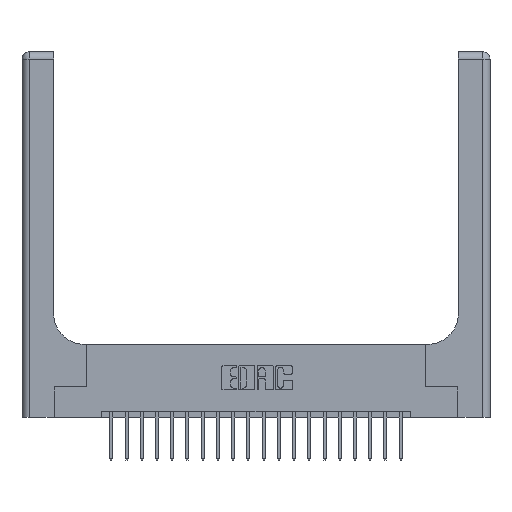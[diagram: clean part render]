
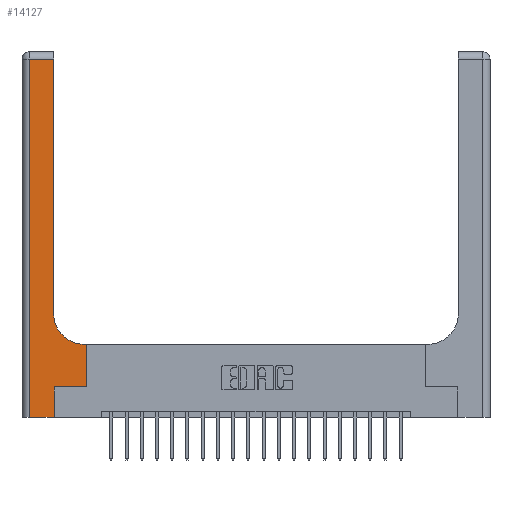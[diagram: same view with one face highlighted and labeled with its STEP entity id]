
A CAD part, top view. The second image highlights one B-rep face of the part: STEP entity #14127.
In plain terms, the highlighted planar face has unit normal (0, 0, 1).
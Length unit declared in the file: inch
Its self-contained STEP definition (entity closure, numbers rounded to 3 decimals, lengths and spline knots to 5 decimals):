
#174 = DIRECTION ( 'NONE',  ( 0., 0., -1. ) ) ;
#272 = ORIENTED_EDGE ( 'NONE', *, *, #4696, .T. ) ;
#410 = VECTOR ( 'NONE', #14561, 39.37008 ) ;
#433 = VERTEX_POINT ( 'NONE', #10053 ) ;
#831 = CARTESIAN_POINT ( 'NONE',  ( 0., 3., 0.37 ) ) ;
#858 = VERTEX_POINT ( 'NONE', #8702 ) ;
#1061 = ORIENTED_EDGE ( 'NONE', *, *, #18924, .T. ) ;
#1114 = CARTESIAN_POINT ( 'NONE',  ( 0.528, 0.25, 0.37 ) ) ;
#1406 = LINE ( 'NONE', #9498, #10198 ) ;
#1642 = EDGE_CURVE ( 'NONE', #13116, #433, #7675, .T. ) ;
#2088 = DIRECTION ( 'NONE',  ( 1., 0., 0. ) ) ;
#2135 = DIRECTION ( 'NONE',  ( 0., -1., 0. ) ) ;
#2728 = VECTOR ( 'NONE', #2088, 39.37008 ) ;
#2782 = VECTOR ( 'NONE', #2135, 39.37008 ) ;
#2784 = VECTOR ( 'NONE', #14777, 39.37008 ) ;
#2836 = CARTESIAN_POINT ( 'NONE',  ( 0.265, 0., 0.37 ) ) ;
#3030 = ORIENTED_EDGE ( 'NONE', *, *, #1642, .T. ) ;
#3148 = VECTOR ( 'NONE', #8522, 39.37008 ) ;
#3284 = VERTEX_POINT ( 'NONE', #2836 ) ;
#3618 = DIRECTION ( 'NONE',  ( -1., 0., 0. ) ) ;
#3716 = LINE ( 'NONE', #10381, #3148 ) ;
#3852 = DIRECTION ( 'NONE',  ( -1., 0., 0. ) ) ;
#4226 = EDGE_CURVE ( 'NONE', #858, #3284, #10407, .T. ) ;
#4638 = ORIENTED_EDGE ( 'NONE', *, *, #8889, .T. ) ;
#4696 = EDGE_CURVE ( 'NONE', #7292, #8135, #3716, .T. ) ;
#4708 = CARTESIAN_POINT ( 'NONE',  ( 0.26, 3., 0.37 ) ) ;
#4794 = CARTESIAN_POINT ( 'NONE',  ( 0.06, 2.94, 0.37 ) ) ;
#4883 = ORIENTED_EDGE ( 'NONE', *, *, #4226, .T. ) ;
#5421 = DIRECTION ( 'NONE',  ( 1., 0., 0. ) ) ;
#5831 = CARTESIAN_POINT ( 'NONE',  ( 0.26, 0.85, 0.37 ) ) ;
#6464 = CARTESIAN_POINT ( 'NONE',  ( 0.265, 0., 0.37 ) ) ;
#7274 = EDGE_LOOP ( 'NONE', ( #13860, #272, #9936, #4883, #1061, #20584, #3030, #10666, #4638 ) ) ;
#7292 = VERTEX_POINT ( 'NONE', #17496 ) ;
#7675 = LINE ( 'NONE', #1114, #10704 ) ;
#7678 = EDGE_CURVE ( 'NONE', #11396, #7292, #21178, .T. ) ;
#8135 = VERTEX_POINT ( 'NONE', #4794 ) ;
#8214 = AXIS2_PLACEMENT_3D ( 'NONE', #831, #14287, #3618 ) ;
#8522 = DIRECTION ( 'NONE',  ( -1., 0., 0. ) ) ;
#8702 = CARTESIAN_POINT ( 'NONE',  ( 0.06, 0., 0.37 ) ) ;
#8889 = EDGE_CURVE ( 'NONE', #16727, #11396, #12022, .T. ) ;
#9256 = FACE_OUTER_BOUND ( 'NONE', #7274, .T. ) ;
#9498 = CARTESIAN_POINT ( 'NONE',  ( 0.265, 0.25, 0.37 ) ) ;
#9524 = CARTESIAN_POINT ( 'NONE',  ( 0.265, 0.25, 0.37 ) ) ;
#9936 = ORIENTED_EDGE ( 'NONE', *, *, #21277, .T. ) ;
#10053 = CARTESIAN_POINT ( 'NONE',  ( 0.528, 0.6, 0.37 ) ) ;
#10198 = VECTOR ( 'NONE', #14319, 39.37008 ) ;
#10381 = CARTESIAN_POINT ( 'NONE',  ( 0., 2.94, 0.37 ) ) ;
#10407 = LINE ( 'NONE', #17017, #2728 ) ;
#10455 = CARTESIAN_POINT ( 'NONE',  ( 0.06, 3., 0.37 ) ) ;
#10607 = AXIS2_PLACEMENT_3D ( 'NONE', #11985, #174, #5421 ) ;
#10666 = ORIENTED_EDGE ( 'NONE', *, *, #14987, .T. ) ;
#10704 = VECTOR ( 'NONE', #16021, 39.37008 ) ;
#11396 = VERTEX_POINT ( 'NONE', #5831 ) ;
#11985 = CARTESIAN_POINT ( 'NONE',  ( 0.51, 0.85, 0.37 ) ) ;
#12022 = CIRCLE ( 'NONE', #10607, 0.25 ) ;
#12416 = LINE ( 'NONE', #10455, #2782 ) ;
#13116 = VERTEX_POINT ( 'NONE', #20294 ) ;
#13860 = ORIENTED_EDGE ( 'NONE', *, *, #7678, .T. ) ;
#14127 = ADVANCED_FACE ( 'NONE', ( #9256 ), #15947, .F. ) ;
#14287 = DIRECTION ( 'NONE',  ( 0., 0., -1. ) ) ;
#14319 = DIRECTION ( 'NONE',  ( 1., 0., 0. ) ) ;
#14543 = CARTESIAN_POINT ( 'NONE',  ( 0.51, 0.6, 0.37 ) ) ;
#14561 = DIRECTION ( 'NONE',  ( 0., 1., 0. ) ) ;
#14671 = LINE ( 'NONE', #6464, #2784 ) ;
#14777 = DIRECTION ( 'NONE',  ( 0., 1., 0. ) ) ;
#14987 = EDGE_CURVE ( 'NONE', #433, #16727, #15350, .T. ) ;
#15149 = VERTEX_POINT ( 'NONE', #9524 ) ;
#15350 = LINE ( 'NONE', #15784, #19109 ) ;
#15784 = CARTESIAN_POINT ( 'NONE',  ( 0.26, 0.6, 0.37 ) ) ;
#15947 = PLANE ( 'NONE',  #8214 ) ;
#16021 = DIRECTION ( 'NONE',  ( 0., 1., 0. ) ) ;
#16727 = VERTEX_POINT ( 'NONE', #14543 ) ;
#17017 = CARTESIAN_POINT ( 'NONE',  ( 0., 0., 0.37 ) ) ;
#17496 = CARTESIAN_POINT ( 'NONE',  ( 0.26, 2.94, 0.37 ) ) ;
#18137 = EDGE_CURVE ( 'NONE', #15149, #13116, #1406, .T. ) ;
#18924 = EDGE_CURVE ( 'NONE', #3284, #15149, #14671, .T. ) ;
#19109 = VECTOR ( 'NONE', #3852, 39.37008 ) ;
#20294 = CARTESIAN_POINT ( 'NONE',  ( 0.528, 0.25, 0.37 ) ) ;
#20584 = ORIENTED_EDGE ( 'NONE', *, *, #18137, .T. ) ;
#21178 = LINE ( 'NONE', #4708, #410 ) ;
#21277 = EDGE_CURVE ( 'NONE', #8135, #858, #12416, .T. ) ;
